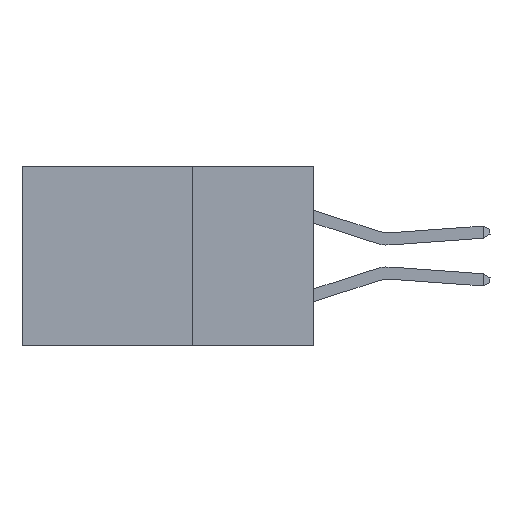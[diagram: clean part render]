
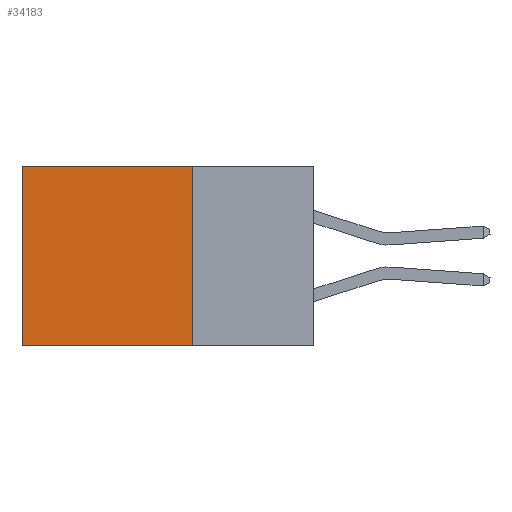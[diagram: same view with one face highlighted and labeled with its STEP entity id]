
A CAD part, left-side view. The second image highlights one B-rep face of the part: STEP entity #34183.
In plain terms, the highlighted planar face has unit normal (-1, 0, 0).
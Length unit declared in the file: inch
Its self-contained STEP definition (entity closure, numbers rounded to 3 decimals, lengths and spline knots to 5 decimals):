
#468 = ORIENTED_EDGE ( 'NONE', *, *, #31576, .T. ) ;
#520 = VECTOR ( 'NONE', #31145, 39.37008 ) ;
#2223 = VERTEX_POINT ( 'NONE', #28376 ) ;
#3663 = ORIENTED_EDGE ( 'NONE', *, *, #12662, .F. ) ;
#4069 = CARTESIAN_POINT ( 'NONE',  ( 0.2875, 0.6, 0. ) ) ;
#5682 = DIRECTION ( 'NONE',  ( 0., 1., 0. ) ) ;
#6564 = ORIENTED_EDGE ( 'NONE', *, *, #29670, .F. ) ;
#7205 = DIRECTION ( 'NONE',  ( 0., 1., 0. ) ) ;
#9733 = CARTESIAN_POINT ( 'NONE',  ( 0.2875, 0.25, 0. ) ) ;
#10897 = LINE ( 'NONE', #25404, #520 ) ;
#11704 = CARTESIAN_POINT ( 'NONE',  ( 0.2875, 0.6, 0. ) ) ;
#11954 = DIRECTION ( 'NONE',  ( 1., 0., 0. ) ) ;
#12662 = EDGE_CURVE ( 'NONE', #31794, #2223, #10897, .T. ) ;
#14052 = CARTESIAN_POINT ( 'NONE',  ( 0.2875, 0.25, 0. ) ) ;
#18286 = CARTESIAN_POINT ( 'NONE',  ( 0.2875, 0.25, -0.37 ) ) ;
#19039 = EDGE_LOOP ( 'NONE', ( #35654, #6564, #3663, #468 ) ) ;
#21338 = LINE ( 'NONE', #4069, #31771 ) ;
#21860 = CARTESIAN_POINT ( 'NONE',  ( 0.2875, 0.6, -0.37 ) ) ;
#22035 = AXIS2_PLACEMENT_3D ( 'NONE', #23489, #11954, #32243 ) ;
#22356 = FACE_OUTER_BOUND ( 'NONE', #19039, .T. ) ;
#22658 = VECTOR ( 'NONE', #5682, 39.37008 ) ;
#23489 = CARTESIAN_POINT ( 'NONE',  ( 0.2875, 0.25, 0. ) ) ;
#24038 = VECTOR ( 'NONE', #7205, 39.37008 ) ;
#24624 = VERTEX_POINT ( 'NONE', #11704 ) ;
#25404 = CARTESIAN_POINT ( 'NONE',  ( 0.2875, 0.25, 0. ) ) ;
#26301 = LINE ( 'NONE', #14052, #22658 ) ;
#27154 = DIRECTION ( 'NONE',  ( 0., 0., -1. ) ) ;
#28376 = CARTESIAN_POINT ( 'NONE',  ( 0.2875, 0.25, -0.37 ) ) ;
#29335 = PLANE ( 'NONE',  #22035 ) ;
#29652 = EDGE_CURVE ( 'NONE', #24624, #32680, #21338, .T. ) ;
#29670 = EDGE_CURVE ( 'NONE', #2223, #32680, #33560, .T. ) ;
#31145 = DIRECTION ( 'NONE',  ( 0., 0., -1. ) ) ;
#31576 = EDGE_CURVE ( 'NONE', #31794, #24624, #26301, .T. ) ;
#31771 = VECTOR ( 'NONE', #27154, 39.37008 ) ;
#31794 = VERTEX_POINT ( 'NONE', #9733 ) ;
#32243 = DIRECTION ( 'NONE',  ( 0., 0., -1. ) ) ;
#32680 = VERTEX_POINT ( 'NONE', #21860 ) ;
#33560 = LINE ( 'NONE', #18286, #24038 ) ;
#34183 = ADVANCED_FACE ( 'NONE', ( #22356 ), #29335, .F. ) ;
#35654 = ORIENTED_EDGE ( 'NONE', *, *, #29652, .T. ) ;
